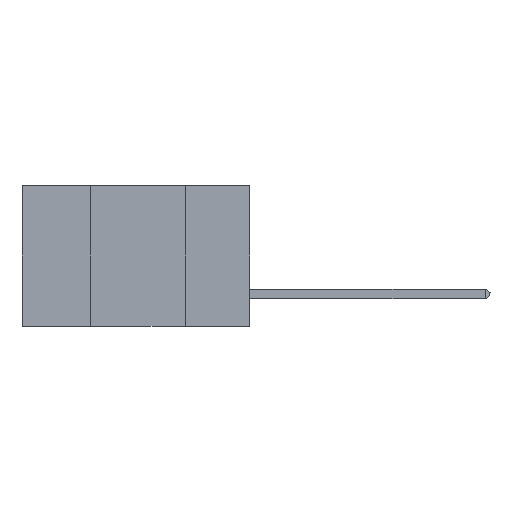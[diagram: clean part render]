
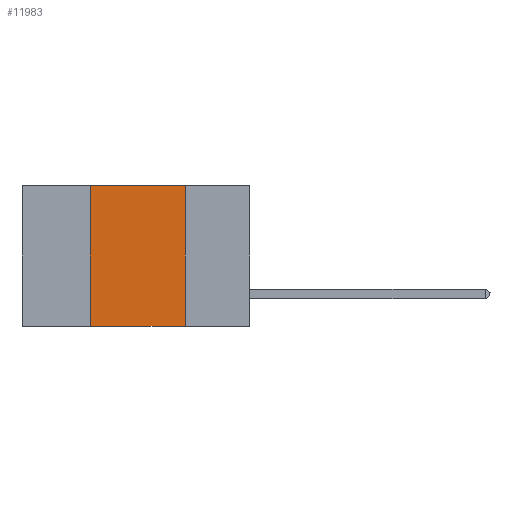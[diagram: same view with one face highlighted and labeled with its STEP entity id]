
A CAD part, left-side view. The second image highlights one B-rep face of the part: STEP entity #11983.
In plain terms, the highlighted planar face has unit normal (-1, 0, 0).
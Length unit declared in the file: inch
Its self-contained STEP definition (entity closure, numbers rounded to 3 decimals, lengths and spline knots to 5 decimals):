
#1456 = EDGE_CURVE ( 'NONE', #7578, #9645, #16837, .T. ) ;
#1612 = PLANE ( 'NONE',  #8788 ) ;
#1623 = VECTOR ( 'NONE', #9105, 39.37008 ) ;
#1870 = VECTOR ( 'NONE', #8372, 39.37008 ) ;
#1978 = ORIENTED_EDGE ( 'NONE', *, *, #11114, .F. ) ;
#2063 = CARTESIAN_POINT ( 'NONE',  ( 0., 0.17, 0. ) ) ;
#3119 = ORIENTED_EDGE ( 'NONE', *, *, #1456, .T. ) ;
#4887 = FACE_OUTER_BOUND ( 'NONE', #12927, .T. ) ;
#5066 = VECTOR ( 'NONE', #7186, 39.37008 ) ;
#5329 = CARTESIAN_POINT ( 'NONE',  ( 0., 0.6, -0.37 ) ) ;
#5559 = LINE ( 'NONE', #2063, #1623 ) ;
#6745 = ORIENTED_EDGE ( 'NONE', *, *, #7661, .F. ) ;
#7092 = VERTEX_POINT ( 'NONE', #7190 ) ;
#7186 = DIRECTION ( 'NONE',  ( 0., 0., 1. ) ) ;
#7190 = CARTESIAN_POINT ( 'NONE',  ( 0., 0.17, 0. ) ) ;
#7411 = CARTESIAN_POINT ( 'NONE',  ( 0., 0.6, 0. ) ) ;
#7578 = VERTEX_POINT ( 'NONE', #11333 ) ;
#7661 = EDGE_CURVE ( 'NONE', #15828, #7092, #17614, .T. ) ;
#8372 = DIRECTION ( 'NONE',  ( 0., -1., 0. ) ) ;
#8788 = AXIS2_PLACEMENT_3D ( 'NONE', #7411, #14125, #11387 ) ;
#8986 = VECTOR ( 'NONE', #16513, 39.37008 ) ;
#9105 = DIRECTION ( 'NONE',  ( 0., 0., -1. ) ) ;
#9645 = VERTEX_POINT ( 'NONE', #15438 ) ;
#9890 = CARTESIAN_POINT ( 'NONE',  ( 0., 0.42, 0. ) ) ;
#10145 = ORIENTED_EDGE ( 'NONE', *, *, #13114, .F. ) ;
#11114 = EDGE_CURVE ( 'NONE', #7092, #9645, #5559, .T. ) ;
#11333 = CARTESIAN_POINT ( 'NONE',  ( 0., 0.42, -0.37 ) ) ;
#11387 = DIRECTION ( 'NONE',  ( 0., 0., -1. ) ) ;
#11918 = CARTESIAN_POINT ( 'NONE',  ( 0., 0.42, 0. ) ) ;
#11983 = ADVANCED_FACE ( 'NONE', ( #4887 ), #1612, .F. ) ;
#12927 = EDGE_LOOP ( 'NONE', ( #1978, #6745, #10145, #3119 ) ) ;
#13114 = EDGE_CURVE ( 'NONE', #7578, #15828, #16201, .T. ) ;
#14125 = DIRECTION ( 'NONE',  ( 1., 0., 0. ) ) ;
#15315 = CARTESIAN_POINT ( 'NONE',  ( 0., 0.6, 0. ) ) ;
#15438 = CARTESIAN_POINT ( 'NONE',  ( 0., 0.17, -0.37 ) ) ;
#15828 = VERTEX_POINT ( 'NONE', #11918 ) ;
#16201 = LINE ( 'NONE', #9890, #5066 ) ;
#16513 = DIRECTION ( 'NONE',  ( 0., -1., 0. ) ) ;
#16837 = LINE ( 'NONE', #5329, #8986 ) ;
#17614 = LINE ( 'NONE', #15315, #1870 ) ;
